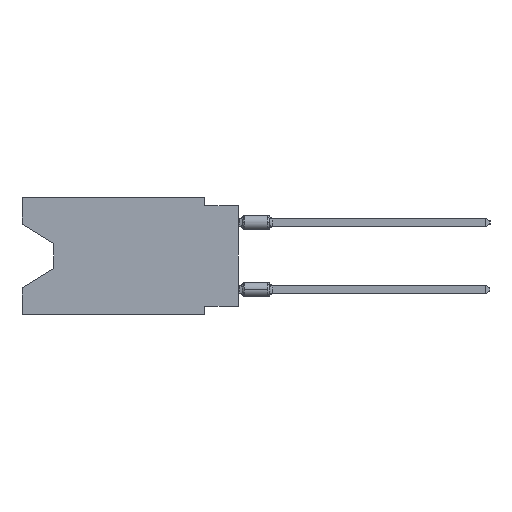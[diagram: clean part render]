
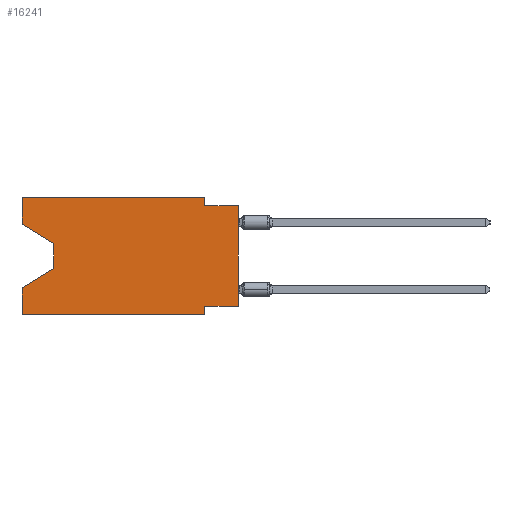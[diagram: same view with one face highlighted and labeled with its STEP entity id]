
A CAD part, left-side view. The second image highlights one B-rep face of the part: STEP entity #16241.
In plain terms, the highlighted planar face has unit normal (-1, 0, 0).
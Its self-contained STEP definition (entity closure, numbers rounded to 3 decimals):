
#525 = VECTOR ( 'NONE', #45035, 1000. ) ;
#1148 = VERTEX_POINT ( 'NONE', #24975 ) ;
#1152 = VERTEX_POINT ( 'NONE', #31841 ) ;
#1295 = CARTESIAN_POINT ( 'NONE',  ( 0., 16.383, -8.89 ) ) ;
#2322 = VECTOR ( 'NONE', #27396, 1000. ) ;
#2674 = LINE ( 'NONE', #18570, #27091 ) ;
#3338 = EDGE_LOOP ( 'NONE', ( #8598, #10152, #11020, #44457, #28484, #6582, #43584, #33260, #33637, #33316, #24020, #39105 ) ) ;
#5936 = VERTEX_POINT ( 'NONE', #13099 ) ;
#6379 = VERTEX_POINT ( 'NONE', #1295 ) ;
#6582 = ORIENTED_EDGE ( 'NONE', *, *, #21044, .F. ) ;
#7618 = LINE ( 'NONE', #21797, #525 ) ;
#8160 = VERTEX_POINT ( 'NONE', #39370 ) ;
#8598 = ORIENTED_EDGE ( 'NONE', *, *, #41401, .T. ) ;
#9174 = VECTOR ( 'NONE', #25413, 1000. ) ;
#9642 = CARTESIAN_POINT ( 'NONE',  ( 0., 16.383, 0. ) ) ;
#10152 = ORIENTED_EDGE ( 'NONE', *, *, #22222, .T. ) ;
#10172 = VERTEX_POINT ( 'NONE', #42162 ) ;
#11020 = ORIENTED_EDGE ( 'NONE', *, *, #33024, .T. ) ;
#11355 = CARTESIAN_POINT ( 'NONE',  ( 0., 16.383, 0. ) ) ;
#12360 = VERTEX_POINT ( 'NONE', #34890 ) ;
#13099 = CARTESIAN_POINT ( 'NONE',  ( 0., 2.54, -8.255 ) ) ;
#13331 = DIRECTION ( 'NONE',  ( 0., 0., 1. ) ) ;
#13560 = DIRECTION ( 'NONE',  ( 0., -1., 0. ) ) ;
#13783 = DIRECTION ( 'NONE',  ( 0., -0.855, -0.519 ) ) ;
#14546 = LINE ( 'NONE', #45368, #42573 ) ;
#14645 = LINE ( 'NONE', #25168, #9174 ) ;
#16039 = DIRECTION ( 'NONE',  ( 1., 0., 0. ) ) ;
#16241 = ADVANCED_FACE ( 'NONE', ( #31947 ), #27068, .F. ) ;
#16454 = EDGE_CURVE ( 'NONE', #8160, #10172, #14546, .T. ) ;
#17010 = DIRECTION ( 'NONE',  ( 0., 0., -1. ) ) ;
#17059 = CARTESIAN_POINT ( 'NONE',  ( 0., 13.97, -5.385 ) ) ;
#17105 = LINE ( 'NONE', #35961, #31169 ) ;
#17529 = LINE ( 'NONE', #32464, #47166 ) ;
#18570 = CARTESIAN_POINT ( 'NONE',  ( 0., 13.97, -3.505 ) ) ;
#19189 = DIRECTION ( 'NONE',  ( 0., -1., 0. ) ) ;
#21044 = EDGE_CURVE ( 'NONE', #5936, #31005, #45994, .T. ) ;
#21285 = VERTEX_POINT ( 'NONE', #42052 ) ;
#21684 = VECTOR ( 'NONE', #30716, 1000. ) ;
#21749 = DIRECTION ( 'NONE',  ( 0., 0., -1. ) ) ;
#21797 = CARTESIAN_POINT ( 'NONE',  ( 0., 0., -8.255 ) ) ;
#22222 = EDGE_CURVE ( 'NONE', #1152, #22501, #2674, .T. ) ;
#22501 = VERTEX_POINT ( 'NONE', #17059 ) ;
#22564 = VECTOR ( 'NONE', #13331, 1000. ) ;
#23024 = EDGE_CURVE ( 'NONE', #21285, #1148, #14645, .T. ) ;
#24020 = ORIENTED_EDGE ( 'NONE', *, *, #16454, .F. ) ;
#24185 = EDGE_CURVE ( 'NONE', #29760, #8160, #45581, .T. ) ;
#24975 = CARTESIAN_POINT ( 'NONE',  ( 0., 0., -0.635 ) ) ;
#25168 = CARTESIAN_POINT ( 'NONE',  ( 0., 0., -0.635 ) ) ;
#25413 = DIRECTION ( 'NONE',  ( 0., -1., 0. ) ) ;
#26524 = DIRECTION ( 'NONE',  ( 0., 0., 1. ) ) ;
#26911 = CARTESIAN_POINT ( 'NONE',  ( 0., 2.54, -8.89 ) ) ;
#27068 = PLANE ( 'NONE',  #32442 ) ;
#27091 = VECTOR ( 'NONE', #21749, 1000. ) ;
#27220 = VECTOR ( 'NONE', #26524, 1000. ) ;
#27396 = DIRECTION ( 'NONE',  ( 0., 0., -1. ) ) ;
#28405 = CARTESIAN_POINT ( 'NONE',  ( 0., 2.54, 0. ) ) ;
#28461 = LINE ( 'NONE', #39983, #42449 ) ;
#28484 = ORIENTED_EDGE ( 'NONE', *, *, #32175, .T. ) ;
#28521 = EDGE_CURVE ( 'NONE', #32294, #5936, #7618, .T. ) ;
#29395 = EDGE_CURVE ( 'NONE', #10172, #21285, #34398, .T. ) ;
#29760 = VERTEX_POINT ( 'NONE', #35224 ) ;
#30631 = EDGE_CURVE ( 'NONE', #6379, #12360, #35842, .T. ) ;
#30716 = DIRECTION ( 'NONE',  ( 0., 0., -1. ) ) ;
#31005 = VERTEX_POINT ( 'NONE', #38895 ) ;
#31169 = VECTOR ( 'NONE', #35714, 1000. ) ;
#31841 = CARTESIAN_POINT ( 'NONE',  ( 0., 13.97, -3.505 ) ) ;
#31947 = FACE_OUTER_BOUND ( 'NONE', #3338, .T. ) ;
#32158 = LINE ( 'NONE', #47068, #45170 ) ;
#32175 = EDGE_CURVE ( 'NONE', #6379, #31005, #32158, .T. ) ;
#32294 = VERTEX_POINT ( 'NONE', #47809 ) ;
#32442 = AXIS2_PLACEMENT_3D ( 'NONE', #42710, #16039, #17010 ) ;
#32464 = CARTESIAN_POINT ( 'NONE',  ( 0., 0., 0. ) ) ;
#33024 = EDGE_CURVE ( 'NONE', #22501, #12360, #17105, .T. ) ;
#33260 = ORIENTED_EDGE ( 'NONE', *, *, #47950, .T. ) ;
#33316 = ORIENTED_EDGE ( 'NONE', *, *, #29395, .F. ) ;
#33637 = ORIENTED_EDGE ( 'NONE', *, *, #23024, .F. ) ;
#34398 = LINE ( 'NONE', #28405, #21684 ) ;
#34890 = CARTESIAN_POINT ( 'NONE',  ( 0., 16.383, -6.852 ) ) ;
#35224 = CARTESIAN_POINT ( 'NONE',  ( 0., 16.383, -2.038 ) ) ;
#35714 = DIRECTION ( 'NONE',  ( 0., 0.855, -0.519 ) ) ;
#35842 = LINE ( 'NONE', #9642, #22564 ) ;
#35961 = CARTESIAN_POINT ( 'NONE',  ( 0., 13.97, -5.385 ) ) ;
#38895 = CARTESIAN_POINT ( 'NONE',  ( 0., 2.54, -8.89 ) ) ;
#39105 = ORIENTED_EDGE ( 'NONE', *, *, #24185, .F. ) ;
#39370 = CARTESIAN_POINT ( 'NONE',  ( 0., 16.383, 0. ) ) ;
#39983 = CARTESIAN_POINT ( 'NONE',  ( 0., 16.383, -2.038 ) ) ;
#41401 = EDGE_CURVE ( 'NONE', #29760, #1152, #28461, .T. ) ;
#42052 = CARTESIAN_POINT ( 'NONE',  ( 0., 2.54, -0.635 ) ) ;
#42162 = CARTESIAN_POINT ( 'NONE',  ( 0., 2.54, 0. ) ) ;
#42449 = VECTOR ( 'NONE', #13783, 1000. ) ;
#42573 = VECTOR ( 'NONE', #19189, 1000. ) ;
#42710 = CARTESIAN_POINT ( 'NONE',  ( 0., 16.383, 0. ) ) ;
#43584 = ORIENTED_EDGE ( 'NONE', *, *, #28521, .F. ) ;
#44457 = ORIENTED_EDGE ( 'NONE', *, *, #30631, .F. ) ;
#45035 = DIRECTION ( 'NONE',  ( 0., 1., 0. ) ) ;
#45170 = VECTOR ( 'NONE', #13560, 1000. ) ;
#45368 = CARTESIAN_POINT ( 'NONE',  ( 0., 16.383, 0. ) ) ;
#45581 = LINE ( 'NONE', #11355, #27220 ) ;
#45994 = LINE ( 'NONE', #26911, #2322 ) ;
#47068 = CARTESIAN_POINT ( 'NONE',  ( 0., 16.383, -8.89 ) ) ;
#47166 = VECTOR ( 'NONE', #47386, 1000. ) ;
#47386 = DIRECTION ( 'NONE',  ( 0., 0., 1. ) ) ;
#47809 = CARTESIAN_POINT ( 'NONE',  ( 0., 0., -8.255 ) ) ;
#47950 = EDGE_CURVE ( 'NONE', #32294, #1148, #17529, .T. ) ;
